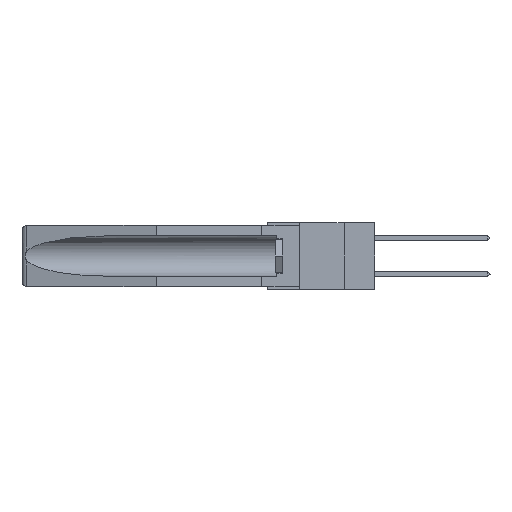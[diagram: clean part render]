
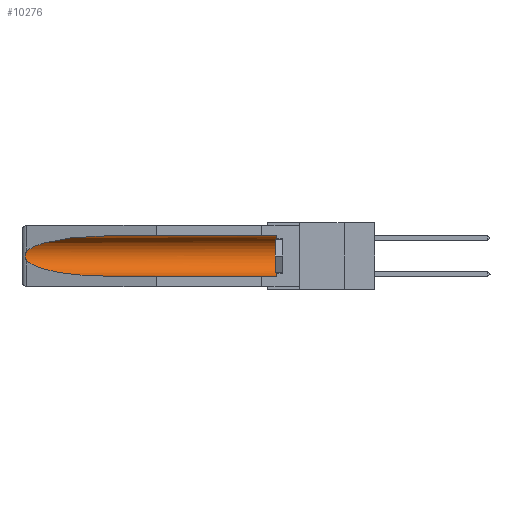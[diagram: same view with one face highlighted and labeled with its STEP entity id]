
A CAD part, left-side view. The second image highlights one B-rep face of the part: STEP entity #10276.
In plain terms, the highlighted cylindrical face has radius 2.857 mm (diameter 5.715 mm), a partial arc.
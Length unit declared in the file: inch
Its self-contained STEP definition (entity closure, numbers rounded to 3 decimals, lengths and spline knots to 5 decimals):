
#1008 = CARTESIAN_POINT ( 'NONE',  ( 0.25451, 1.48313, -0.09465 ) ) ;
#1553 = AXIS2_PLACEMENT_3D ( 'NONE', #2135, #2374, #15860 ) ;
#1761 = ORIENTED_EDGE ( 'NONE', *, *, #21684, .T. ) ;
#2135 = CARTESIAN_POINT ( 'NONE',  ( 0.155, 0.126, -0.1715 ) ) ;
#2150 = DIRECTION ( 'NONE',  ( 0., 0., 1. ) ) ;
#2374 = DIRECTION ( 'NONE',  ( 0., -1., 0. ) ) ;
#2982 = CARTESIAN_POINT ( 'NONE',  ( 0.26537, 1.52718, -0.14972 ) ) ;
#3490 = FACE_OUTER_BOUND ( 'NONE', #25074, .T. ) ;
#3526 = CARTESIAN_POINT ( 'NONE',  ( 0.155, 1.07973, -0.284 ) ) ;
#4103 = VERTEX_POINT ( 'NONE', #9048 ) ;
#5724 = CARTESIAN_POINT ( 'NONE',  ( 0.26655, 1.53094, -0.18657 ) ) ;
#5814 = CARTESIAN_POINT ( 'NONE',  ( 0.155, -0.30754, -0.059 ) ) ;
#5974 = CARTESIAN_POINT ( 'NONE',  ( 0.2675, 1.53308, -0.17534 ) ) ;
#5988 = AXIS2_PLACEMENT_3D ( 'NONE', #10076, #17839, #2150 ) ;
#7802 = CARTESIAN_POINT ( 'NONE',  ( 0.26654, 1.53092, -0.15636 ) ) ;
#7854 = ORIENTED_EDGE ( 'NONE', *, *, #18289, .T. ) ;
#7909 = EDGE_CURVE ( 'NONE', #10872, #21716, #20420, .T. ) ;
#8886 = CARTESIAN_POINT ( 'NONE',  ( 0.26537, 1.52718, -0.14972 ) ) ;
#9048 = CARTESIAN_POINT ( 'NONE',  ( 0.155, 0.126, -0.059 ) ) ;
#9796 = CARTESIAN_POINT ( 'NONE',  ( 0.2673, 1.53269, -0.17917 ) ) ;
#9819 = DIRECTION ( 'NONE',  ( 0., 1., 0. ) ) ;
#10076 = CARTESIAN_POINT ( 'NONE',  ( 0.155, -0.30754, -0.1715 ) ) ;
#10276 = ADVANCED_FACE ( 'NONE', ( #3490 ), #15149, .F. ) ;
#10872 = VERTEX_POINT ( 'NONE', #18095 ) ;
#11434 = CARTESIAN_POINT ( 'NONE',  ( 0.21114, 1.30732, -0.284 ) ) ;
#11780 = CARTESIAN_POINT ( 'NONE',  ( 0.155, -0.30754, -0.284 ) ) ;
#11994 = CARTESIAN_POINT ( 'NONE',  ( 0.26537, 1.52718, -0.19328 ) ) ;
#12145 =( BOUNDED_CURVE ( )  B_SPLINE_CURVE ( 3, ( #15091, #23032, #11434, #3526 ),
 .UNSPECIFIED., .F., .F. ) 
 B_SPLINE_CURVE_WITH_KNOTS ( ( 4, 4 ),
 ( 0.1948, 1.5708 ),
 .UNSPECIFIED. ) 
 CURVE ( )  GEOMETRIC_REPRESENTATION_ITEM ( )  RATIONAL_B_SPLINE_CURVE ( ( 1., 0.848, 0.848, 1. ) ) 
 REPRESENTATION_ITEM ( '' )  );
#12953 = ORIENTED_EDGE ( 'NONE', *, *, #7909, .F. ) ;
#13481 = VERTEX_POINT ( 'NONE', #8886 ) ;
#13663 = LINE ( 'NONE', #5814, #20757 ) ;
#13844 = ORIENTED_EDGE ( 'NONE', *, *, #14028, .T. ) ;
#13985 = CIRCLE ( 'NONE', #1553, 0.1125 ) ;
#14028 = EDGE_CURVE ( 'NONE', #23772, #21716, #12145, .T. ) ;
#14564 = VECTOR ( 'NONE', #9819, 39.37008 ) ;
#15091 = CARTESIAN_POINT ( 'NONE',  ( 0.26537, 1.52718, -0.19328 ) ) ;
#15149 = CYLINDRICAL_SURFACE ( 'NONE', #5988, 0.1125 ) ;
#15294 = CARTESIAN_POINT ( 'NONE',  ( 0.26537, 1.52718, -0.19328 ) ) ;
#15860 = DIRECTION ( 'NONE',  ( 0., 0., 1. ) ) ;
#15896 =( BOUNDED_CURVE ( )  B_SPLINE_CURVE ( 3, ( #20605, #20687, #1008, #2982 ),
 .UNSPECIFIED., .F., .F. ) 
 B_SPLINE_CURVE_WITH_KNOTS ( ( 4, 4 ),
 ( 4.71239, 6.08839 ),
 .UNSPECIFIED. ) 
 CURVE ( )  GEOMETRIC_REPRESENTATION_ITEM ( )  RATIONAL_B_SPLINE_CURVE ( ( 1., 0.848, 0.848, 1. ) ) 
 REPRESENTATION_ITEM ( '' )  );
#16754 = ORIENTED_EDGE ( 'NONE', *, *, #24952, .T. ) ;
#17545 = CARTESIAN_POINT ( 'NONE',  ( 0.2675, 1.53308, -0.16763 ) ) ;
#17724 = CARTESIAN_POINT ( 'NONE',  ( 0.26537, 1.52718, -0.14972 ) ) ;
#17839 = DIRECTION ( 'NONE',  ( 0., 1., 0. ) ) ;
#18095 = CARTESIAN_POINT ( 'NONE',  ( 0.155, 0.126, -0.284 ) ) ;
#18289 = EDGE_CURVE ( 'NONE', #13481, #23772, #24745, .T. ) ;
#18322 = EDGE_CURVE ( 'NONE', #4103, #20578, #13663, .T. ) ;
#18996 = CARTESIAN_POINT ( 'NONE',  ( 0.155, 1.07973, -0.059 ) ) ;
#19575 = CARTESIAN_POINT ( 'NONE',  ( 0.26597, 1.52961, -0.15275 ) ) ;
#20084 = CARTESIAN_POINT ( 'NONE',  ( 0.155, 1.07973, -0.284 ) ) ;
#20420 = LINE ( 'NONE', #11780, #14564 ) ;
#20578 = VERTEX_POINT ( 'NONE', #18996 ) ;
#20605 = CARTESIAN_POINT ( 'NONE',  ( 0.155, 1.07973, -0.059 ) ) ;
#20687 = CARTESIAN_POINT ( 'NONE',  ( 0.21114, 1.30732, -0.059 ) ) ;
#20757 = VECTOR ( 'NONE', #21625, 39.37008 ) ;
#20836 = ORIENTED_EDGE ( 'NONE', *, *, #18322, .T. ) ;
#21625 = DIRECTION ( 'NONE',  ( 0., 1., 0. ) ) ;
#21684 = EDGE_CURVE ( 'NONE', #10872, #4103, #13985, .T. ) ;
#21716 = VERTEX_POINT ( 'NONE', #20084 ) ;
#23032 = CARTESIAN_POINT ( 'NONE',  ( 0.25451, 1.48313, -0.24835 ) ) ;
#23444 = CARTESIAN_POINT ( 'NONE',  ( 0.2673, 1.5327, -0.16383 ) ) ;
#23539 = CARTESIAN_POINT ( 'NONE',  ( 0.26597, 1.5296, -0.19026 ) ) ;
#23772 = VERTEX_POINT ( 'NONE', #15294 ) ;
#24745 = B_SPLINE_CURVE_WITH_KNOTS ( 'NONE', 3,
 ( #17724, #19575, #7802, #23444, #17545, #5974, #9796, #5724, #23539, #11994 ),
 .UNSPECIFIED., .F., .F.,
 ( 4, 2, 2, 2, 4 ),
 ( 0., 0.00029, 0.00058, 0.00087, 0.00117 ),
 .UNSPECIFIED. ) ;
#24952 = EDGE_CURVE ( 'NONE', #20578, #13481, #15896, .T. ) ;
#25074 = EDGE_LOOP ( 'NONE', ( #16754, #7854, #13844, #12953, #1761, #20836 ) ) ;
